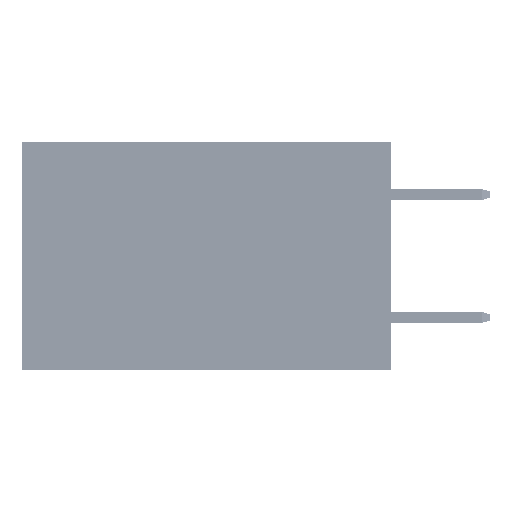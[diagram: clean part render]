
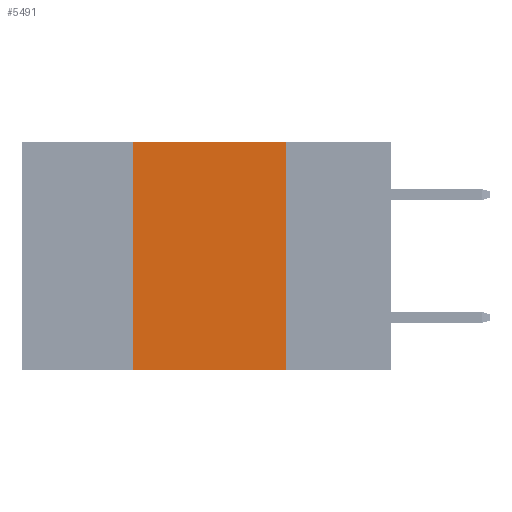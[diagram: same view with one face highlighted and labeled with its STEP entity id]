
A CAD part, left-side view. The second image highlights one B-rep face of the part: STEP entity #5491.
In plain terms, the highlighted planar face has unit normal (-1, 0, 0).
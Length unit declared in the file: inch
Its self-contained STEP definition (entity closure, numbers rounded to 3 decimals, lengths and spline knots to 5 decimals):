
#30 = VECTOR ( 'NONE', #45883, 39.37008 ) ;
#1924 = FACE_OUTER_BOUND ( 'NONE', #34646, .T. ) ;
#4630 = CARTESIAN_POINT ( 'NONE',  ( 0., 0.6, 0. ) ) ;
#5491 = ADVANCED_FACE ( 'NONE', ( #1924 ), #12325, .F. ) ;
#5711 = AXIS2_PLACEMENT_3D ( 'NONE', #4630, #8771, #16123 ) ;
#6919 = CARTESIAN_POINT ( 'NONE',  ( 0., 0.17, 0. ) ) ;
#8571 = LINE ( 'NONE', #10799, #50987 ) ;
#8707 = DIRECTION ( 'NONE',  ( 0., -1., 0. ) ) ;
#8771 = DIRECTION ( 'NONE',  ( 1., 0., 0. ) ) ;
#8889 = VERTEX_POINT ( 'NONE', #42314 ) ;
#10799 = CARTESIAN_POINT ( 'NONE',  ( 0., 0.17, 0. ) ) ;
#12133 = VERTEX_POINT ( 'NONE', #25803 ) ;
#12153 = DIRECTION ( 'NONE',  ( 0., 0., -1. ) ) ;
#12325 = PLANE ( 'NONE',  #5711 ) ;
#13912 = EDGE_CURVE ( 'NONE', #47112, #48302, #34961, .T. ) ;
#16123 = DIRECTION ( 'NONE',  ( 0., 0., -1. ) ) ;
#19179 = EDGE_CURVE ( 'NONE', #12133, #47112, #21859, .T. ) ;
#21859 = LINE ( 'NONE', #36564, #30 ) ;
#22351 = EDGE_CURVE ( 'NONE', #48302, #8889, #8571, .T. ) ;
#22532 = CARTESIAN_POINT ( 'NONE',  ( 0., 0.42, 0. ) ) ;
#23520 = ORIENTED_EDGE ( 'NONE', *, *, #22351, .F. ) ;
#25803 = CARTESIAN_POINT ( 'NONE',  ( 0., 0.42, -0.37 ) ) ;
#28242 = VECTOR ( 'NONE', #8707, 39.37008 ) ;
#30547 = ORIENTED_EDGE ( 'NONE', *, *, #13912, .F. ) ;
#34221 = ORIENTED_EDGE ( 'NONE', *, *, #38049, .T. ) ;
#34646 = EDGE_LOOP ( 'NONE', ( #23520, #30547, #40077, #34221 ) ) ;
#34687 = DIRECTION ( 'NONE',  ( 0., -1., 0. ) ) ;
#34961 = LINE ( 'NONE', #47076, #49046 ) ;
#36564 = CARTESIAN_POINT ( 'NONE',  ( 0., 0.42, 0. ) ) ;
#38049 = EDGE_CURVE ( 'NONE', #12133, #8889, #42982, .T. ) ;
#40077 = ORIENTED_EDGE ( 'NONE', *, *, #19179, .F. ) ;
#42314 = CARTESIAN_POINT ( 'NONE',  ( 0., 0.17, -0.37 ) ) ;
#42982 = LINE ( 'NONE', #49653, #28242 ) ;
#45883 = DIRECTION ( 'NONE',  ( 0., 0., 1. ) ) ;
#47076 = CARTESIAN_POINT ( 'NONE',  ( 0., 0.6, 0. ) ) ;
#47112 = VERTEX_POINT ( 'NONE', #22532 ) ;
#48302 = VERTEX_POINT ( 'NONE', #6919 ) ;
#49046 = VECTOR ( 'NONE', #34687, 39.37008 ) ;
#49653 = CARTESIAN_POINT ( 'NONE',  ( 0., 0.6, -0.37 ) ) ;
#50987 = VECTOR ( 'NONE', #12153, 39.37008 ) ;
